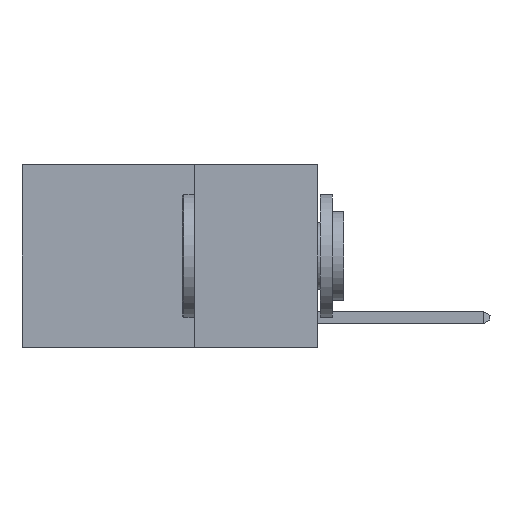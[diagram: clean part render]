
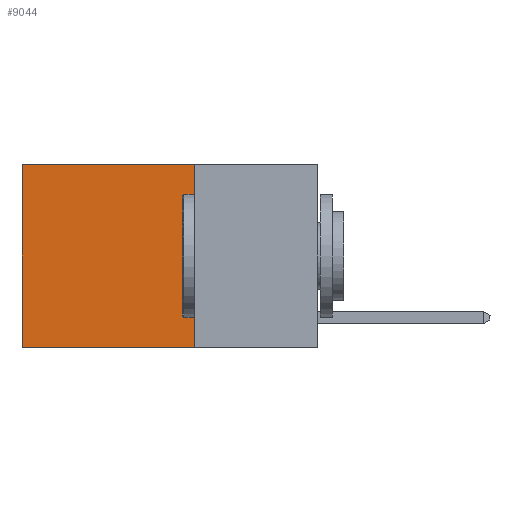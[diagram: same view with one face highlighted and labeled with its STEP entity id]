
A CAD part, left-side view. The second image highlights one B-rep face of the part: STEP entity #9044.
In plain terms, the highlighted planar face has unit normal (-1, 0, 0).
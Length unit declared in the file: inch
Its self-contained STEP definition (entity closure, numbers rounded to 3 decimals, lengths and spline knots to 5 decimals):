
#663 = DIRECTION ( 'NONE',  ( 1., 0., 0. ) ) ;
#940 = VERTEX_POINT ( 'NONE', #13954 ) ;
#1143 = LINE ( 'NONE', #18274, #11836 ) ;
#2823 = DIRECTION ( 'NONE',  ( 0., 1., 0. ) ) ;
#6138 = ORIENTED_EDGE ( 'NONE', *, *, #17911, .F. ) ;
#7930 = FACE_OUTER_BOUND ( 'NONE', #23659, .T. ) ;
#7955 = LINE ( 'NONE', #8605, #23890 ) ;
#8605 = CARTESIAN_POINT ( 'NONE',  ( 0.2625, 0.25, 0. ) ) ;
#9044 = ADVANCED_FACE ( 'NONE', ( #7930 ), #22094, .F. ) ;
#10153 = LINE ( 'NONE', #13569, #15677 ) ;
#10209 = CARTESIAN_POINT ( 'NONE',  ( 0.2625, 0.25, 0. ) ) ;
#11804 = VERTEX_POINT ( 'NONE', #20796 ) ;
#11836 = VECTOR ( 'NONE', #2823, 39.37008 ) ;
#12009 = VERTEX_POINT ( 'NONE', #18112 ) ;
#12128 = EDGE_CURVE ( 'NONE', #12009, #11804, #1143, .T. ) ;
#12904 = ORIENTED_EDGE ( 'NONE', *, *, #17829, .T. ) ;
#13569 = CARTESIAN_POINT ( 'NONE',  ( 0.2625, 0.6, 0. ) ) ;
#13954 = CARTESIAN_POINT ( 'NONE',  ( 0.2625, 0.6, 0. ) ) ;
#14160 = DIRECTION ( 'NONE',  ( 0., 0., -1. ) ) ;
#15677 = VECTOR ( 'NONE', #21345, 39.37008 ) ;
#17344 = EDGE_CURVE ( 'NONE', #22831, #940, #23610, .T. ) ;
#17520 = DIRECTION ( 'NONE',  ( 0., 1., 0. ) ) ;
#17829 = EDGE_CURVE ( 'NONE', #940, #11804, #10153, .T. ) ;
#17911 = EDGE_CURVE ( 'NONE', #22831, #12009, #7955, .T. ) ;
#18112 = CARTESIAN_POINT ( 'NONE',  ( 0.2625, 0.25, -0.37 ) ) ;
#18274 = CARTESIAN_POINT ( 'NONE',  ( 0.2625, 0.25, -0.37 ) ) ;
#19112 = ORIENTED_EDGE ( 'NONE', *, *, #12128, .F. ) ;
#19340 = VECTOR ( 'NONE', #17520, 39.37008 ) ;
#19443 = ORIENTED_EDGE ( 'NONE', *, *, #17344, .T. ) ;
#19780 = AXIS2_PLACEMENT_3D ( 'NONE', #10209, #663, #14160 ) ;
#20316 = DIRECTION ( 'NONE',  ( 0., 0., -1. ) ) ;
#20772 = CARTESIAN_POINT ( 'NONE',  ( 0.2625, 0.25, 0. ) ) ;
#20796 = CARTESIAN_POINT ( 'NONE',  ( 0.2625, 0.6, -0.37 ) ) ;
#21345 = DIRECTION ( 'NONE',  ( 0., 0., -1. ) ) ;
#22094 = PLANE ( 'NONE',  #19780 ) ;
#22831 = VERTEX_POINT ( 'NONE', #20772 ) ;
#23610 = LINE ( 'NONE', #23747, #19340 ) ;
#23659 = EDGE_LOOP ( 'NONE', ( #12904, #19112, #6138, #19443 ) ) ;
#23747 = CARTESIAN_POINT ( 'NONE',  ( 0.2625, 0.25, 0. ) ) ;
#23890 = VECTOR ( 'NONE', #20316, 39.37008 ) ;
